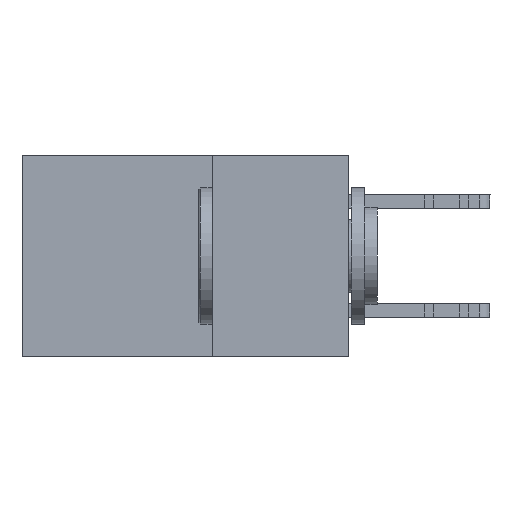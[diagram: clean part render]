
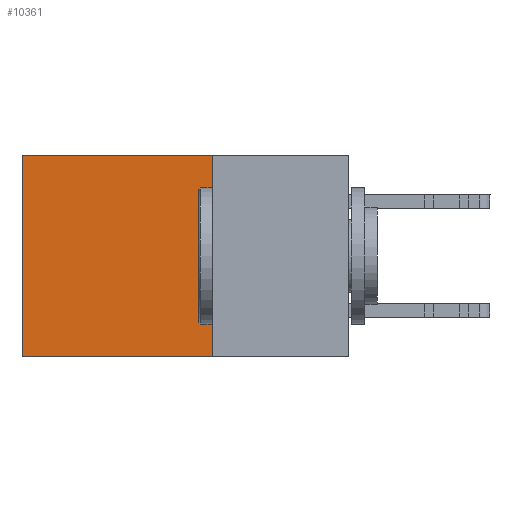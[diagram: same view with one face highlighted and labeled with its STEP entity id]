
A CAD part, left-side view. The second image highlights one B-rep face of the part: STEP entity #10361.
In plain terms, the highlighted planar face has unit normal (-1, 0, 0).
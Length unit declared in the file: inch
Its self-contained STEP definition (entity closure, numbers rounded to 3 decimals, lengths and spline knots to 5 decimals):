
#137 = ORIENTED_EDGE ( 'NONE', *, *, #27028, .F. ) ;
#1226 = AXIS2_PLACEMENT_3D ( 'NONE', #1611, #7839, #19502 ) ;
#1611 = CARTESIAN_POINT ( 'NONE',  ( 0.298, 0.25, 0. ) ) ;
#2021 = CARTESIAN_POINT ( 'NONE',  ( 0.298, 0.25, 0. ) ) ;
#3035 = DIRECTION ( 'NONE',  ( 0., 0., -1. ) ) ;
#3063 = EDGE_CURVE ( 'NONE', #21364, #18586, #25246, .T. ) ;
#4096 = VERTEX_POINT ( 'NONE', #4646 ) ;
#4646 = CARTESIAN_POINT ( 'NONE',  ( 0.298, 0.25, -0.37 ) ) ;
#6100 = VERTEX_POINT ( 'NONE', #13923 ) ;
#7839 = DIRECTION ( 'NONE',  ( 1., 0., 0. ) ) ;
#9786 = VECTOR ( 'NONE', #12011, 39.37008 ) ;
#9980 = CARTESIAN_POINT ( 'NONE',  ( 0.298, 0.25, 0. ) ) ;
#10028 = VECTOR ( 'NONE', #14262, 39.37008 ) ;
#10253 = PLANE ( 'NONE',  #1226 ) ;
#10361 = ADVANCED_FACE ( 'NONE', ( #22373 ), #10253, .F. ) ;
#11574 = CARTESIAN_POINT ( 'NONE',  ( 0.298, 0.25, 0. ) ) ;
#12011 = DIRECTION ( 'NONE',  ( 0., 1., 0. ) ) ;
#12045 = VECTOR ( 'NONE', #23094, 39.37008 ) ;
#12804 = EDGE_CURVE ( 'NONE', #18586, #6100, #14406, .T. ) ;
#13923 = CARTESIAN_POINT ( 'NONE',  ( 0.298, 0.6, -0.37 ) ) ;
#14262 = DIRECTION ( 'NONE',  ( 0., 0., -1. ) ) ;
#14406 = LINE ( 'NONE', #18963, #10028 ) ;
#17789 = EDGE_LOOP ( 'NONE', ( #28404, #25642, #137, #27103 ) ) ;
#18586 = VERTEX_POINT ( 'NONE', #27309 ) ;
#18963 = CARTESIAN_POINT ( 'NONE',  ( 0.298, 0.6, 0. ) ) ;
#19131 = CARTESIAN_POINT ( 'NONE',  ( 0.298, 0.25, -0.37 ) ) ;
#19236 = LINE ( 'NONE', #9980, #21441 ) ;
#19502 = DIRECTION ( 'NONE',  ( 0., 0., -1. ) ) ;
#21364 = VERTEX_POINT ( 'NONE', #2021 ) ;
#21441 = VECTOR ( 'NONE', #3035, 39.37008 ) ;
#22373 = FACE_OUTER_BOUND ( 'NONE', #17789, .T. ) ;
#23094 = DIRECTION ( 'NONE',  ( 0., 1., 0. ) ) ;
#25246 = LINE ( 'NONE', #11574, #12045 ) ;
#25642 = ORIENTED_EDGE ( 'NONE', *, *, #27800, .F. ) ;
#27028 = EDGE_CURVE ( 'NONE', #21364, #4096, #19236, .T. ) ;
#27103 = ORIENTED_EDGE ( 'NONE', *, *, #3063, .T. ) ;
#27309 = CARTESIAN_POINT ( 'NONE',  ( 0.298, 0.6, 0. ) ) ;
#27800 = EDGE_CURVE ( 'NONE', #4096, #6100, #28098, .T. ) ;
#28098 = LINE ( 'NONE', #19131, #9786 ) ;
#28404 = ORIENTED_EDGE ( 'NONE', *, *, #12804, .T. ) ;
